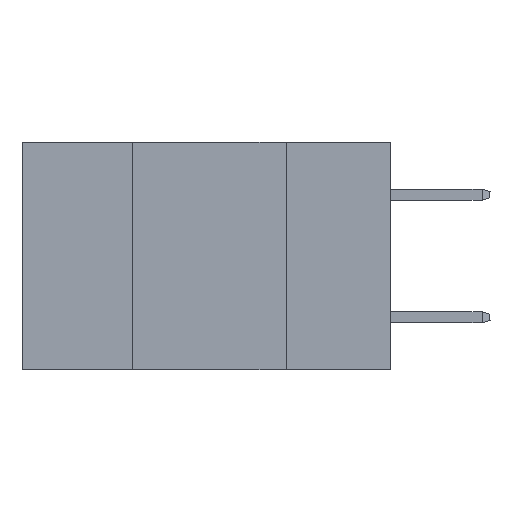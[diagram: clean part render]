
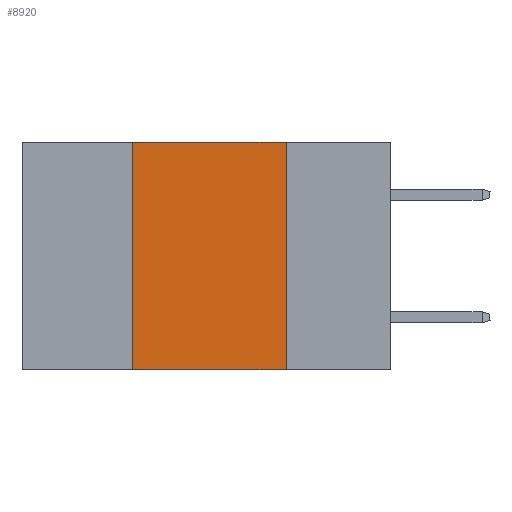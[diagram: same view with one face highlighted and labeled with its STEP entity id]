
A CAD part, left-side view. The second image highlights one B-rep face of the part: STEP entity #8920.
In plain terms, the highlighted planar face has unit normal (-1, 0, 0).
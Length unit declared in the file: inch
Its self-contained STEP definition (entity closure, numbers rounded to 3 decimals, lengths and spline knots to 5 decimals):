
#1327 = EDGE_CURVE ( 'NONE', #38327, #8544, #35454, .T. ) ;
#2462 = CARTESIAN_POINT ( 'NONE',  ( 0., 0.17, -0.37 ) ) ;
#3030 = CARTESIAN_POINT ( 'NONE',  ( 0., 0.42, 0. ) ) ;
#3181 = VERTEX_POINT ( 'NONE', #32475 ) ;
#3959 = EDGE_CURVE ( 'NONE', #8544, #5094, #29434, .T. ) ;
#5094 = VERTEX_POINT ( 'NONE', #2462 ) ;
#5398 = VECTOR ( 'NONE', #6513, 39.37008 ) ;
#6466 = DIRECTION ( 'NONE',  ( 1., 0., 0. ) ) ;
#6513 = DIRECTION ( 'NONE',  ( 0., 0., -1. ) ) ;
#6565 = DIRECTION ( 'NONE',  ( 0., 0., 1. ) ) ;
#7354 = DIRECTION ( 'NONE',  ( 0., -1., 0. ) ) ;
#8544 = VERTEX_POINT ( 'NONE', #11240 ) ;
#8920 = ADVANCED_FACE ( 'NONE', ( #29545 ), #36618, .F. ) ;
#9507 = DIRECTION ( 'NONE',  ( 0., 0., -1. ) ) ;
#11240 = CARTESIAN_POINT ( 'NONE',  ( 0., 0.17, 0. ) ) ;
#15107 = VECTOR ( 'NONE', #33741, 39.37008 ) ;
#15338 = ORIENTED_EDGE ( 'NONE', *, *, #3959, .F. ) ;
#16018 = CARTESIAN_POINT ( 'NONE',  ( 0., 0.42, 0. ) ) ;
#18992 = CARTESIAN_POINT ( 'NONE',  ( 0., 0.6, -0.37 ) ) ;
#24543 = LINE ( 'NONE', #18992, #15107 ) ;
#27505 = ORIENTED_EDGE ( 'NONE', *, *, #34161, .T. ) ;
#29434 = LINE ( 'NONE', #36406, #5398 ) ;
#29545 = FACE_OUTER_BOUND ( 'NONE', #36601, .T. ) ;
#30567 = CARTESIAN_POINT ( 'NONE',  ( 0., 0.6, 0. ) ) ;
#31300 = CARTESIAN_POINT ( 'NONE',  ( 0., 0.6, 0. ) ) ;
#32475 = CARTESIAN_POINT ( 'NONE',  ( 0., 0.42, -0.37 ) ) ;
#33741 = DIRECTION ( 'NONE',  ( 0., -1., 0. ) ) ;
#34161 = EDGE_CURVE ( 'NONE', #3181, #5094, #24543, .T. ) ;
#35302 = EDGE_CURVE ( 'NONE', #3181, #38327, #37636, .T. ) ;
#35454 = LINE ( 'NONE', #31300, #37803 ) ;
#36253 = AXIS2_PLACEMENT_3D ( 'NONE', #30567, #6466, #9507 ) ;
#36406 = CARTESIAN_POINT ( 'NONE',  ( 0., 0.17, 0. ) ) ;
#36601 = EDGE_LOOP ( 'NONE', ( #15338, #36866, #38540, #27505 ) ) ;
#36618 = PLANE ( 'NONE',  #36253 ) ;
#36866 = ORIENTED_EDGE ( 'NONE', *, *, #1327, .F. ) ;
#37185 = VECTOR ( 'NONE', #6565, 39.37008 ) ;
#37636 = LINE ( 'NONE', #3030, #37185 ) ;
#37803 = VECTOR ( 'NONE', #7354, 39.37008 ) ;
#38327 = VERTEX_POINT ( 'NONE', #16018 ) ;
#38540 = ORIENTED_EDGE ( 'NONE', *, *, #35302, .F. ) ;
